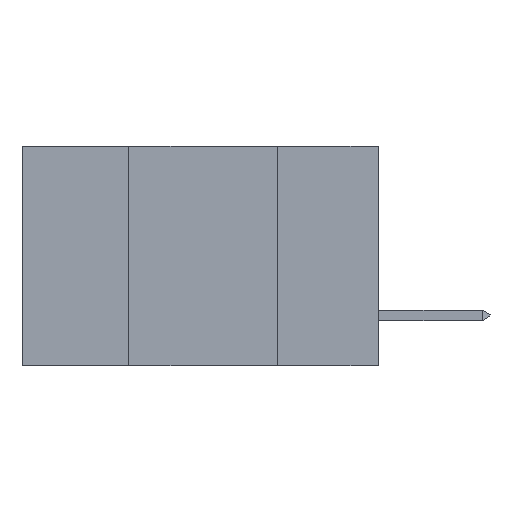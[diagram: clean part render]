
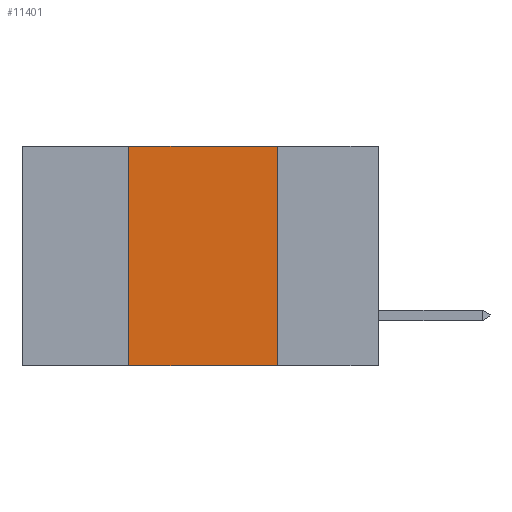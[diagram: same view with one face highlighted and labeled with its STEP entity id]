
A CAD part, left-side view. The second image highlights one B-rep face of the part: STEP entity #11401.
In plain terms, the highlighted planar face has unit normal (-1, 0, 0).
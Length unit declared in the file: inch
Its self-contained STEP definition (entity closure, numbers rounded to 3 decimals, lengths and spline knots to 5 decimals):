
#2289 = PLANE ( 'NONE',  #4795 ) ;
#2333 = CARTESIAN_POINT ( 'NONE',  ( 0., 0.42, 0. ) ) ;
#2478 = VECTOR ( 'NONE', #22771, 39.37008 ) ;
#2803 = CARTESIAN_POINT ( 'NONE',  ( 0., 0.17, -0.37 ) ) ;
#3174 = EDGE_LOOP ( 'NONE', ( #11282, #9945, #18141, #8918 ) ) ;
#3285 = DIRECTION ( 'NONE',  ( 0., -1., 0. ) ) ;
#3335 = LINE ( 'NONE', #19625, #7020 ) ;
#3889 = VERTEX_POINT ( 'NONE', #15951 ) ;
#4309 = DIRECTION ( 'NONE',  ( 0., 0., -1. ) ) ;
#4795 = AXIS2_PLACEMENT_3D ( 'NONE', #21317, #18670, #4309 ) ;
#6821 = DIRECTION ( 'NONE',  ( 0., 0., -1. ) ) ;
#7020 = VECTOR ( 'NONE', #19539, 39.37008 ) ;
#7755 = CARTESIAN_POINT ( 'NONE',  ( 0., 0.42, 0. ) ) ;
#8562 = EDGE_CURVE ( 'NONE', #3889, #20934, #21137, .T. ) ;
#8918 = ORIENTED_EDGE ( 'NONE', *, *, #8562, .T. ) ;
#8961 = CARTESIAN_POINT ( 'NONE',  ( 0., 0.6, -0.37 ) ) ;
#9945 = ORIENTED_EDGE ( 'NONE', *, *, #22457, .F. ) ;
#10031 = FACE_OUTER_BOUND ( 'NONE', #3174, .T. ) ;
#10877 = LINE ( 'NONE', #23825, #27302 ) ;
#11282 = ORIENTED_EDGE ( 'NONE', *, *, #16633, .F. ) ;
#11401 = ADVANCED_FACE ( 'NONE', ( #10031 ), #2289, .F. ) ;
#15443 = VECTOR ( 'NONE', #3285, 39.37008 ) ;
#15951 = CARTESIAN_POINT ( 'NONE',  ( 0., 0.42, -0.37 ) ) ;
#16633 = EDGE_CURVE ( 'NONE', #25648, #20934, #10877, .T. ) ;
#17314 = VERTEX_POINT ( 'NONE', #2333 ) ;
#18141 = ORIENTED_EDGE ( 'NONE', *, *, #20001, .F. ) ;
#18670 = DIRECTION ( 'NONE',  ( 1., 0., 0. ) ) ;
#19539 = DIRECTION ( 'NONE',  ( 0., -1., 0. ) ) ;
#19582 = LINE ( 'NONE', #7755, #2478 ) ;
#19625 = CARTESIAN_POINT ( 'NONE',  ( 0., 0.6, 0. ) ) ;
#20001 = EDGE_CURVE ( 'NONE', #3889, #17314, #19582, .T. ) ;
#20934 = VERTEX_POINT ( 'NONE', #2803 ) ;
#21137 = LINE ( 'NONE', #8961, #15443 ) ;
#21317 = CARTESIAN_POINT ( 'NONE',  ( 0., 0.6, 0. ) ) ;
#21462 = CARTESIAN_POINT ( 'NONE',  ( 0., 0.17, 0. ) ) ;
#22457 = EDGE_CURVE ( 'NONE', #17314, #25648, #3335, .T. ) ;
#22771 = DIRECTION ( 'NONE',  ( 0., 0., 1. ) ) ;
#23825 = CARTESIAN_POINT ( 'NONE',  ( 0., 0.17, 0. ) ) ;
#25648 = VERTEX_POINT ( 'NONE', #21462 ) ;
#27302 = VECTOR ( 'NONE', #6821, 39.37008 ) ;
